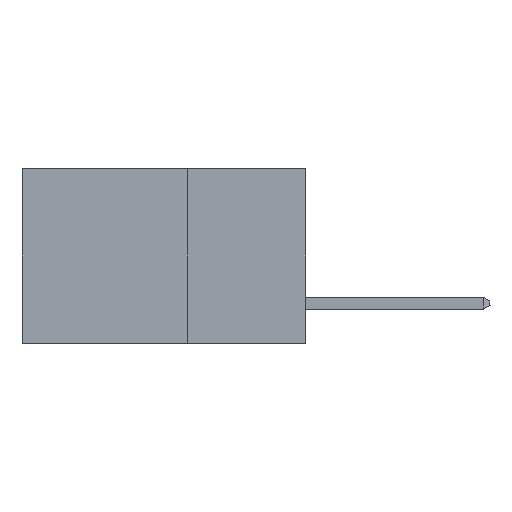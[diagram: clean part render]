
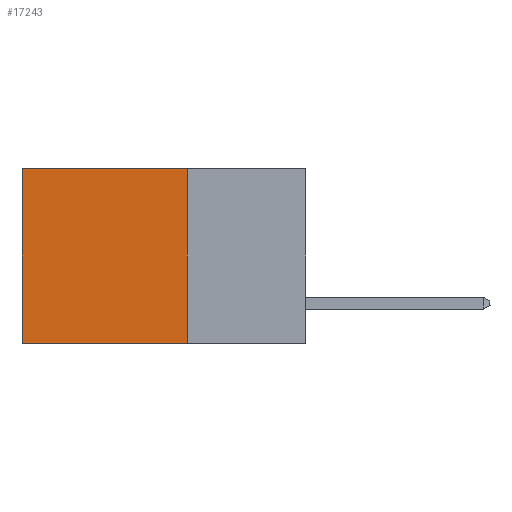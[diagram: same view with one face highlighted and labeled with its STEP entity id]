
A CAD part, left-side view. The second image highlights one B-rep face of the part: STEP entity #17243.
In plain terms, the highlighted planar face has unit normal (-1, 0, 0).
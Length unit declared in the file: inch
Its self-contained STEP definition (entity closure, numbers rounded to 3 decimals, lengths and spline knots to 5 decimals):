
#27 = CARTESIAN_POINT ( 'NONE',  ( 0.298, 0.25, -0.37 ) ) ;
#463 = VERTEX_POINT ( 'NONE', #2324 ) ;
#598 = EDGE_CURVE ( 'NONE', #463, #3234, #27798, .T. ) ;
#1187 = ORIENTED_EDGE ( 'NONE', *, *, #598, .T. ) ;
#1337 = ORIENTED_EDGE ( 'NONE', *, *, #28080, .F. ) ;
#2324 = CARTESIAN_POINT ( 'NONE',  ( 0.298, 0.25, 0. ) ) ;
#2721 = CARTESIAN_POINT ( 'NONE',  ( 0.298, 0.25, 0. ) ) ;
#2751 = CARTESIAN_POINT ( 'NONE',  ( 0.298, 0.6, 0. ) ) ;
#3234 = VERTEX_POINT ( 'NONE', #2751 ) ;
#3418 = FACE_OUTER_BOUND ( 'NONE', #24150, .T. ) ;
#3643 = ORIENTED_EDGE ( 'NONE', *, *, #24883, .T. ) ;
#6279 = DIRECTION ( 'NONE',  ( 0., 0., -1. ) ) ;
#7251 = DIRECTION ( 'NONE',  ( 0., 1., 0. ) ) ;
#8500 = CARTESIAN_POINT ( 'NONE',  ( 0.298, 0.6, 0. ) ) ;
#9309 = VECTOR ( 'NONE', #7251, 39.37008 ) ;
#10169 = CARTESIAN_POINT ( 'NONE',  ( 0.298, 0.25, 0. ) ) ;
#11052 = CARTESIAN_POINT ( 'NONE',  ( 0.298, 0.25, 0. ) ) ;
#16348 = VECTOR ( 'NONE', #27622, 39.37008 ) ;
#17006 = DIRECTION ( 'NONE',  ( 0., 0., -1. ) ) ;
#17243 = ADVANCED_FACE ( 'NONE', ( #3418 ), #19346, .F. ) ;
#18740 = VERTEX_POINT ( 'NONE', #27 ) ;
#19346 = PLANE ( 'NONE',  #28273 ) ;
#22449 = DIRECTION ( 'NONE',  ( 0., 0., -1. ) ) ;
#22597 = LINE ( 'NONE', #23159, #16348 ) ;
#23159 = CARTESIAN_POINT ( 'NONE',  ( 0.298, 0.25, -0.37 ) ) ;
#23642 = VECTOR ( 'NONE', #6279, 39.37008 ) ;
#24150 = EDGE_LOOP ( 'NONE', ( #3643, #1337, #27037, #1187 ) ) ;
#24883 = EDGE_CURVE ( 'NONE', #3234, #26087, #28444, .T. ) ;
#26087 = VERTEX_POINT ( 'NONE', #28083 ) ;
#26607 = DIRECTION ( 'NONE',  ( 1., 0., 0. ) ) ;
#27037 = ORIENTED_EDGE ( 'NONE', *, *, #29256, .F. ) ;
#27622 = DIRECTION ( 'NONE',  ( 0., 1., 0. ) ) ;
#27798 = LINE ( 'NONE', #2721, #9309 ) ;
#28080 = EDGE_CURVE ( 'NONE', #18740, #26087, #22597, .T. ) ;
#28083 = CARTESIAN_POINT ( 'NONE',  ( 0.298, 0.6, -0.37 ) ) ;
#28273 = AXIS2_PLACEMENT_3D ( 'NONE', #10169, #26607, #17006 ) ;
#28444 = LINE ( 'NONE', #8500, #29197 ) ;
#29197 = VECTOR ( 'NONE', #22449, 39.37008 ) ;
#29256 = EDGE_CURVE ( 'NONE', #463, #18740, #29943, .T. ) ;
#29943 = LINE ( 'NONE', #11052, #23642 ) ;
